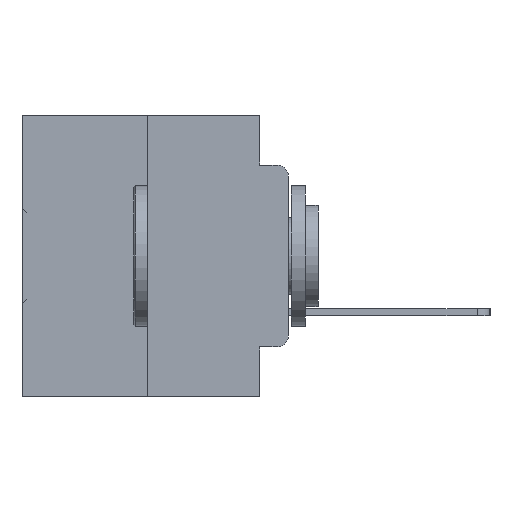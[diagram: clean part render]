
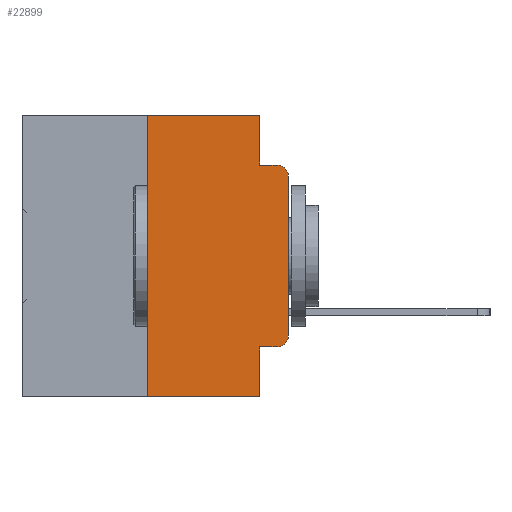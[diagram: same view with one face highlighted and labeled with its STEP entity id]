
A CAD part, left-side view. The second image highlights one B-rep face of the part: STEP entity #22899.
In plain terms, the highlighted planar face has unit normal (-1, 0, 0).
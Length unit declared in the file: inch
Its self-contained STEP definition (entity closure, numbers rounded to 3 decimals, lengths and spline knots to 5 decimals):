
#89 = DIRECTION ( 'NONE',  ( -1., 0., 0. ) ) ;
#338 = FACE_OUTER_BOUND ( 'NONE', #28622, .T. ) ;
#972 = EDGE_CURVE ( 'NONE', #26955, #24761, #5148, .T. ) ;
#1361 = VECTOR ( 'NONE', #8926, 39.37008 ) ;
#1583 = EDGE_CURVE ( 'NONE', #30843, #13791, #18493, .T. ) ;
#1624 = CARTESIAN_POINT ( 'NONE',  ( 0., 0.25, 0. ) ) ;
#2385 = LINE ( 'NONE', #18545, #22211 ) ;
#2600 = ORIENTED_EDGE ( 'NONE', *, *, #7062, .F. ) ;
#3457 = DIRECTION ( 'NONE',  ( -1., 0., 0. ) ) ;
#4728 = ORIENTED_EDGE ( 'NONE', *, *, #19697, .F. ) ;
#5148 = LINE ( 'NONE', #13610, #25717 ) ;
#5240 = EDGE_CURVE ( 'NONE', #30843, #9766, #9854, .T. ) ;
#6111 = CARTESIAN_POINT ( 'NONE',  ( 0., 0., -0.1085 ) ) ;
#6223 = CARTESIAN_POINT ( 'NONE',  ( 0., 0.051, -0.0885 ) ) ;
#6754 = CIRCLE ( 'NONE', #21154, 0.02 ) ;
#7062 = EDGE_CURVE ( 'NONE', #25786, #26955, #14349, .T. ) ;
#7163 = VECTOR ( 'NONE', #9698, 39.37008 ) ;
#7311 = DIRECTION ( 'NONE',  ( 0., 0., -1. ) ) ;
#7357 = VECTOR ( 'NONE', #29520, 39.37008 ) ;
#7647 = VERTEX_POINT ( 'NONE', #27335 ) ;
#8134 = CIRCLE ( 'NONE', #29948, 0.02 ) ;
#8926 = DIRECTION ( 'NONE',  ( 0., -1., 0. ) ) ;
#8956 = ORIENTED_EDGE ( 'NONE', *, *, #28567, .T. ) ;
#9698 = DIRECTION ( 'NONE',  ( 0., 0., 1. ) ) ;
#9766 = VERTEX_POINT ( 'NONE', #28121 ) ;
#9816 = CARTESIAN_POINT ( 'NONE',  ( 0., 0.051, 0. ) ) ;
#9854 = LINE ( 'NONE', #9816, #22432 ) ;
#10692 = EDGE_CURVE ( 'NONE', #24761, #7647, #22495, .T. ) ;
#10882 = CARTESIAN_POINT ( 'NONE',  ( 0., 0.051, 0. ) ) ;
#13087 = ORIENTED_EDGE ( 'NONE', *, *, #1583, .T. ) ;
#13329 = VERTEX_POINT ( 'NONE', #21386 ) ;
#13610 = CARTESIAN_POINT ( 'NONE',  ( 0., 0.473, 0. ) ) ;
#13791 = VERTEX_POINT ( 'NONE', #31261 ) ;
#14349 = LINE ( 'NONE', #1624, #7163 ) ;
#14857 = CARTESIAN_POINT ( 'NONE',  ( 0., 0., -0.3915 ) ) ;
#16261 = CARTESIAN_POINT ( 'NONE',  ( 0., 0.02, -0.3915 ) ) ;
#17623 = VECTOR ( 'NONE', #27908, 39.37008 ) ;
#17677 = ORIENTED_EDGE ( 'NONE', *, *, #10692, .F. ) ;
#18042 = CARTESIAN_POINT ( 'NONE',  ( 0., 0.473, 0. ) ) ;
#18493 = LINE ( 'NONE', #27572, #17623 ) ;
#18545 = CARTESIAN_POINT ( 'NONE',  ( 0., 0., 0. ) ) ;
#18948 = ORIENTED_EDGE ( 'NONE', *, *, #30969, .T. ) ;
#18989 = DIRECTION ( 'NONE',  ( 0., 0., -1. ) ) ;
#19250 = ORIENTED_EDGE ( 'NONE', *, *, #5240, .F. ) ;
#19317 = DIRECTION ( 'NONE',  ( 0., -1., 0. ) ) ;
#19656 = CARTESIAN_POINT ( 'NONE',  ( 0., 0.02, -0.1085 ) ) ;
#19697 = EDGE_CURVE ( 'NONE', #7647, #13329, #30709, .T. ) ;
#19770 = ORIENTED_EDGE ( 'NONE', *, *, #972, .F. ) ;
#21089 = CARTESIAN_POINT ( 'NONE',  ( 0., 0.051, -0.4115 ) ) ;
#21108 = VERTEX_POINT ( 'NONE', #14857 ) ;
#21154 = AXIS2_PLACEMENT_3D ( 'NONE', #19656, #3457, #22325 ) ;
#21239 = DIRECTION ( 'NONE',  ( 0., 0., 1. ) ) ;
#21290 = LINE ( 'NONE', #29519, #27482 ) ;
#21386 = CARTESIAN_POINT ( 'NONE',  ( 0., 0.02, -0.0885 ) ) ;
#21476 = EDGE_CURVE ( 'NONE', #23251, #13329, #6754, .T. ) ;
#22211 = VECTOR ( 'NONE', #21239, 39.37008 ) ;
#22285 = ORIENTED_EDGE ( 'NONE', *, *, #24840, .T. ) ;
#22325 = DIRECTION ( 'NONE',  ( 0., 0., -1. ) ) ;
#22432 = VECTOR ( 'NONE', #25848, 39.37008 ) ;
#22495 = LINE ( 'NONE', #10882, #7357 ) ;
#22899 = ADVANCED_FACE ( 'NONE', ( #338 ), #28597, .F. ) ;
#23251 = VERTEX_POINT ( 'NONE', #6111 ) ;
#23396 = DIRECTION ( 'NONE',  ( 1., 0., 0. ) ) ;
#23738 = CARTESIAN_POINT ( 'NONE',  ( 0., 0.051, 0. ) ) ;
#24761 = VERTEX_POINT ( 'NONE', #23738 ) ;
#24840 = EDGE_CURVE ( 'NONE', #25786, #9766, #21290, .T. ) ;
#25548 = CARTESIAN_POINT ( 'NONE',  ( 0., 0.25, -0.5 ) ) ;
#25717 = VECTOR ( 'NONE', #19317, 39.37008 ) ;
#25786 = VERTEX_POINT ( 'NONE', #25548 ) ;
#25848 = DIRECTION ( 'NONE',  ( 0., 0., -1. ) ) ;
#26047 = ORIENTED_EDGE ( 'NONE', *, *, #21476, .T. ) ;
#26955 = VERTEX_POINT ( 'NONE', #31210 ) ;
#27335 = CARTESIAN_POINT ( 'NONE',  ( 0., 0.051, -0.0885 ) ) ;
#27371 = AXIS2_PLACEMENT_3D ( 'NONE', #18042, #23396, #7311 ) ;
#27482 = VECTOR ( 'NONE', #32147, 39.37008 ) ;
#27572 = CARTESIAN_POINT ( 'NONE',  ( 0., 0.051, -0.4115 ) ) ;
#27908 = DIRECTION ( 'NONE',  ( 0., -1., 0. ) ) ;
#28121 = CARTESIAN_POINT ( 'NONE',  ( 0., 0.051, -0.5 ) ) ;
#28567 = EDGE_CURVE ( 'NONE', #21108, #23251, #2385, .T. ) ;
#28597 = PLANE ( 'NONE',  #27371 ) ;
#28622 = EDGE_LOOP ( 'NONE', ( #8956, #26047, #4728, #17677, #19770, #2600, #22285, #19250, #13087, #18948 ) ) ;
#29519 = CARTESIAN_POINT ( 'NONE',  ( 0., 0.473, -0.5 ) ) ;
#29520 = DIRECTION ( 'NONE',  ( 0., 0., -1. ) ) ;
#29948 = AXIS2_PLACEMENT_3D ( 'NONE', #16261, #89, #18989 ) ;
#30709 = LINE ( 'NONE', #6223, #1361 ) ;
#30843 = VERTEX_POINT ( 'NONE', #21089 ) ;
#30969 = EDGE_CURVE ( 'NONE', #13791, #21108, #8134, .T. ) ;
#31210 = CARTESIAN_POINT ( 'NONE',  ( 0., 0.25, 0. ) ) ;
#31261 = CARTESIAN_POINT ( 'NONE',  ( 0., 0.02, -0.4115 ) ) ;
#32147 = DIRECTION ( 'NONE',  ( 0., -1., 0. ) ) ;
